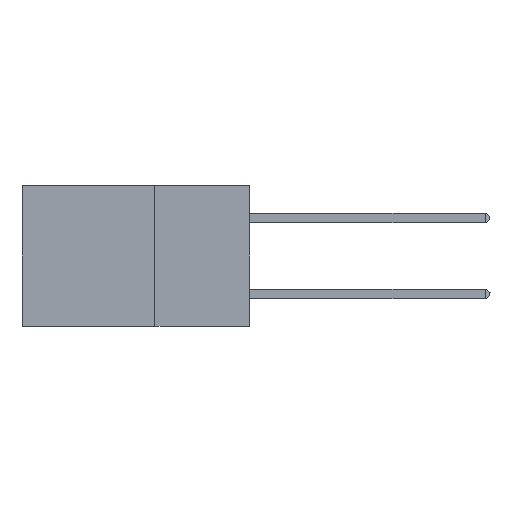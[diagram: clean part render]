
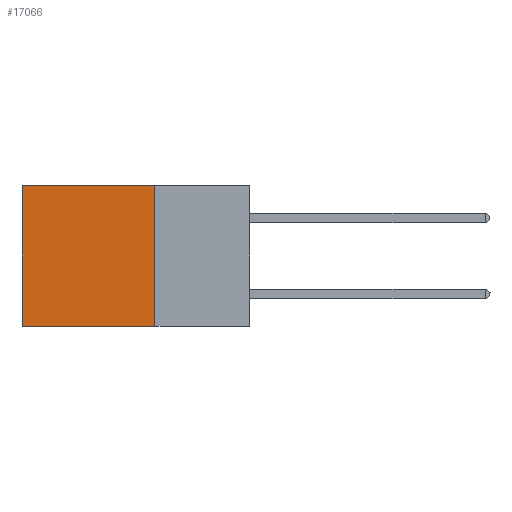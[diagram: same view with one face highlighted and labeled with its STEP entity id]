
A CAD part, left-side view. The second image highlights one B-rep face of the part: STEP entity #17066.
In plain terms, the highlighted planar face has unit normal (-1, 0, 0).
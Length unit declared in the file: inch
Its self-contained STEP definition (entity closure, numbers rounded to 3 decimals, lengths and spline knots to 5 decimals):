
#1966 = VERTEX_POINT ( 'NONE', #18735 ) ;
#2814 = ORIENTED_EDGE ( 'NONE', *, *, #8267, .T. ) ;
#3216 = VECTOR ( 'NONE', #22957, 39.37008 ) ;
#5609 = VECTOR ( 'NONE', #17282, 39.37008 ) ;
#6180 = EDGE_LOOP ( 'NONE', ( #2814, #19316, #9654, #7238 ) ) ;
#6556 = CARTESIAN_POINT ( 'NONE',  ( 0.2875, 0.25, 0. ) ) ;
#7238 = ORIENTED_EDGE ( 'NONE', *, *, #8578, .T. ) ;
#7612 = DIRECTION ( 'NONE',  ( 0., 1., 0. ) ) ;
#8267 = EDGE_CURVE ( 'NONE', #16569, #11240, #20822, .T. ) ;
#8578 = EDGE_CURVE ( 'NONE', #23254, #16569, #14241, .T. ) ;
#9356 = VECTOR ( 'NONE', #7612, 39.37008 ) ;
#9654 = ORIENTED_EDGE ( 'NONE', *, *, #23168, .F. ) ;
#9981 = CARTESIAN_POINT ( 'NONE',  ( 0.2875, 0.6, 0. ) ) ;
#10471 = AXIS2_PLACEMENT_3D ( 'NONE', #10992, #14438, #21977 ) ;
#10992 = CARTESIAN_POINT ( 'NONE',  ( 0.2875, 0.25, 0. ) ) ;
#11240 = VERTEX_POINT ( 'NONE', #14630 ) ;
#12837 = CARTESIAN_POINT ( 'NONE',  ( 0.2875, 0.25, 0. ) ) ;
#13151 = FACE_OUTER_BOUND ( 'NONE', #6180, .T. ) ;
#14241 = LINE ( 'NONE', #12837, #9356 ) ;
#14438 = DIRECTION ( 'NONE',  ( 1., 0., 0. ) ) ;
#14537 = LINE ( 'NONE', #23722, #22298 ) ;
#14630 = CARTESIAN_POINT ( 'NONE',  ( 0.2875, 0.6, -0.37 ) ) ;
#15238 = CARTESIAN_POINT ( 'NONE',  ( 0.2875, 0.25, 0. ) ) ;
#15455 = CARTESIAN_POINT ( 'NONE',  ( 0.2875, 0.6, 0. ) ) ;
#16402 = PLANE ( 'NONE',  #10471 ) ;
#16569 = VERTEX_POINT ( 'NONE', #9981 ) ;
#16838 = DIRECTION ( 'NONE',  ( 0., 1., 0. ) ) ;
#17066 = ADVANCED_FACE ( 'NONE', ( #13151 ), #16402, .F. ) ;
#17282 = DIRECTION ( 'NONE',  ( 0., 0., -1. ) ) ;
#17908 = EDGE_CURVE ( 'NONE', #1966, #11240, #14537, .T. ) ;
#18735 = CARTESIAN_POINT ( 'NONE',  ( 0.2875, 0.25, -0.37 ) ) ;
#19316 = ORIENTED_EDGE ( 'NONE', *, *, #17908, .F. ) ;
#20822 = LINE ( 'NONE', #15455, #5609 ) ;
#21977 = DIRECTION ( 'NONE',  ( 0., 0., -1. ) ) ;
#22168 = LINE ( 'NONE', #15238, #3216 ) ;
#22298 = VECTOR ( 'NONE', #16838, 39.37008 ) ;
#22957 = DIRECTION ( 'NONE',  ( 0., 0., -1. ) ) ;
#23168 = EDGE_CURVE ( 'NONE', #23254, #1966, #22168, .T. ) ;
#23254 = VERTEX_POINT ( 'NONE', #6556 ) ;
#23722 = CARTESIAN_POINT ( 'NONE',  ( 0.2875, 0.25, -0.37 ) ) ;
